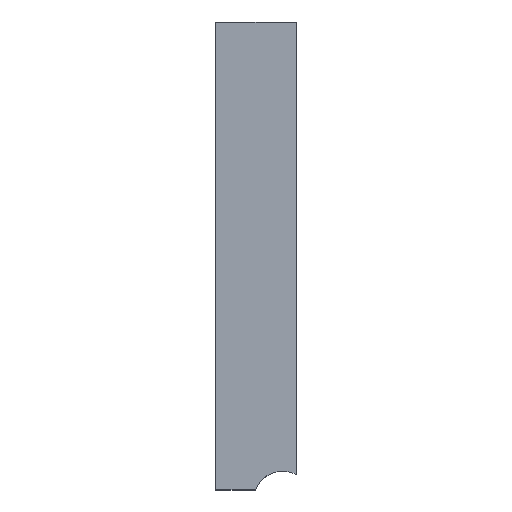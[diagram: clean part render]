
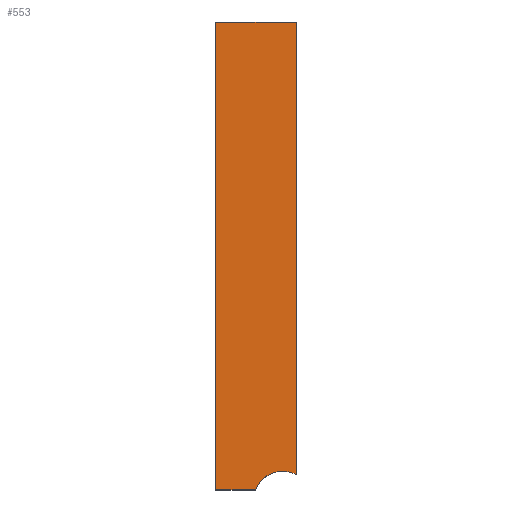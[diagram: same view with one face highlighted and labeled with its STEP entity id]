
A CAD part, top view. The second image highlights one B-rep face of the part: STEP entity #553.
In plain terms, the highlighted planar face has unit normal (0, 0, 1).
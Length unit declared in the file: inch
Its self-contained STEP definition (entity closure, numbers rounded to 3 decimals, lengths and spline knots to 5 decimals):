
#5 = CARTESIAN_POINT ( 'NONE',  ( 1.37795, 0.26319, 0. ) ) ;
#59 = CARTESIAN_POINT ( 'NONE',  ( 0.68, 0., 0. ) ) ;
#100 = LINE ( 'NONE', #5, #506 ) ;
#128 = EDGE_CURVE ( 'NONE', #757, #295, #100, .T. ) ;
#147 = DIRECTION ( 'NONE',  ( 0., 0., -1. ) ) ;
#161 = CIRCLE ( 'NONE', #796, 0.5 ) ;
#207 = DIRECTION ( 'NONE',  ( 1., 0., 0. ) ) ;
#208 = LINE ( 'NONE', #355, #725 ) ;
#242 = ORIENTED_EDGE ( 'NONE', *, *, #514, .T. ) ;
#267 = CARTESIAN_POINT ( 'NONE',  ( 0., 0., 0. ) ) ;
#273 = PLANE ( 'NONE',  #366 ) ;
#295 = VERTEX_POINT ( 'NONE', #607 ) ;
#319 = EDGE_CURVE ( 'NONE', #457, #707, #936, .T. ) ;
#355 = CARTESIAN_POINT ( 'NONE',  ( 0., 8., 0. ) ) ;
#359 = CARTESIAN_POINT ( 'NONE',  ( 0., 8., 0. ) ) ;
#364 = VECTOR ( 'NONE', #391, 39.37008 ) ;
#366 = AXIS2_PLACEMENT_3D ( 'NONE', #415, #629, #207 ) ;
#391 = DIRECTION ( 'NONE',  ( 0., 1., 0. ) ) ;
#415 = CARTESIAN_POINT ( 'NONE',  ( 0., 0., 0. ) ) ;
#431 = ORIENTED_EDGE ( 'NONE', *, *, #701, .T. ) ;
#457 = VERTEX_POINT ( 'NONE', #836 ) ;
#467 = CARTESIAN_POINT ( 'NONE',  ( 0., 0., 0. ) ) ;
#489 = FACE_OUTER_BOUND ( 'NONE', #858, .T. ) ;
#506 = VECTOR ( 'NONE', #515, 39.37008 ) ;
#514 = EDGE_CURVE ( 'NONE', #457, #567, #896, .T. ) ;
#515 = DIRECTION ( 'NONE',  ( 0., 1., 0. ) ) ;
#553 = ADVANCED_FACE ( 'NONE', ( #489 ), #273, .T. ) ;
#567 = VERTEX_POINT ( 'NONE', #59 ) ;
#577 = ORIENTED_EDGE ( 'NONE', *, *, #319, .F. ) ;
#580 = CARTESIAN_POINT ( 'NONE',  ( 1.14648, -0.18, 0. ) ) ;
#607 = CARTESIAN_POINT ( 'NONE',  ( 1.37795, 8., 0. ) ) ;
#629 = DIRECTION ( 'NONE',  ( 0., 0., 1. ) ) ;
#648 = DIRECTION ( 'NONE',  ( -0.933, 0.36, 0. ) ) ;
#650 = CARTESIAN_POINT ( 'NONE',  ( 1.37795, 0.26319, 0. ) ) ;
#692 = EDGE_CURVE ( 'NONE', #707, #295, #208, .T. ) ;
#697 = VECTOR ( 'NONE', #923, 39.37008 ) ;
#701 = EDGE_CURVE ( 'NONE', #567, #757, #161, .T. ) ;
#707 = VERTEX_POINT ( 'NONE', #359 ) ;
#710 = DIRECTION ( 'NONE',  ( 1., 0., 0. ) ) ;
#725 = VECTOR ( 'NONE', #710, 39.37008 ) ;
#757 = VERTEX_POINT ( 'NONE', #650 ) ;
#796 = AXIS2_PLACEMENT_3D ( 'NONE', #580, #147, #648 ) ;
#836 = CARTESIAN_POINT ( 'NONE',  ( 0., 0., 0. ) ) ;
#858 = EDGE_LOOP ( 'NONE', ( #919, #924, #577, #242, #431 ) ) ;
#896 = LINE ( 'NONE', #267, #697 ) ;
#919 = ORIENTED_EDGE ( 'NONE', *, *, #128, .T. ) ;
#923 = DIRECTION ( 'NONE',  ( 1., 0., 0. ) ) ;
#924 = ORIENTED_EDGE ( 'NONE', *, *, #692, .F. ) ;
#936 = LINE ( 'NONE', #467, #364 ) ;
